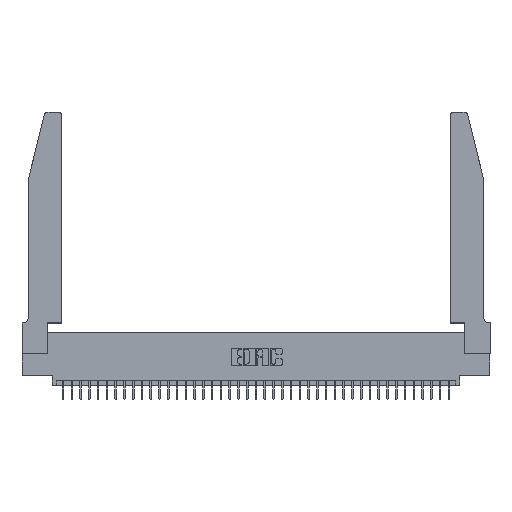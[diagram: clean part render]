
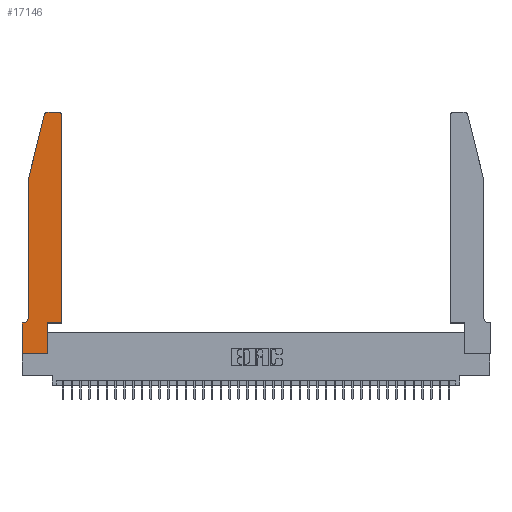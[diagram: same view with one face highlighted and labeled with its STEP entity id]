
A CAD part, top view. The second image highlights one B-rep face of the part: STEP entity #17146.
In plain terms, the highlighted planar face has unit normal (0, 0, 1).
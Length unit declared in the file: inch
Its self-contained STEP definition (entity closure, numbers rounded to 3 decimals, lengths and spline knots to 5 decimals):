
#1031 = EDGE_CURVE ( 'NONE', #5443, #14733, #7668, .T. ) ;
#1682 = ORIENTED_EDGE ( 'NONE', *, *, #4806, .T. ) ;
#1684 = DIRECTION ( 'NONE',  ( -1., 0., 0. ) ) ;
#2002 = AXIS2_PLACEMENT_3D ( 'NONE', #31600, #16380, #37752 ) ;
#3697 = CARTESIAN_POINT ( 'NONE',  ( 0.4505, 2.72, 0.37 ) ) ;
#4222 = CIRCLE ( 'NONE', #11011, 0.03 ) ;
#4514 = VERTEX_POINT ( 'NONE', #37365 ) ;
#4765 = EDGE_CURVE ( 'NONE', #20373, #31066, #15623, .T. ) ;
#4806 = EDGE_CURVE ( 'NONE', #36230, #12499, #21822, .T. ) ;
#4904 = CARTESIAN_POINT ( 'NONE',  ( 0.2865, 0.35, 0.37 ) ) ;
#4975 = CARTESIAN_POINT ( 'NONE',  ( 0.0055, 0.35, 0.37 ) ) ;
#5207 = DIRECTION ( 'NONE',  ( 0., -1., 0. ) ) ;
#5320 = LINE ( 'NONE', #6671, #22719 ) ;
#5443 = VERTEX_POINT ( 'NONE', #14033 ) ;
#5752 = EDGE_CURVE ( 'NONE', #4514, #20373, #5320, .T. ) ;
#5785 = AXIS2_PLACEMENT_3D ( 'NONE', #25825, #28760, #36079 ) ;
#6391 = DIRECTION ( 'NONE',  ( 0., 0., 1. ) ) ;
#6575 = ORIENTED_EDGE ( 'NONE', *, *, #12706, .T. ) ;
#6606 = LINE ( 'NONE', #24565, #22051 ) ;
#6671 = CARTESIAN_POINT ( 'NONE',  ( 0.2865, 0.35, 0.37 ) ) ;
#6973 = AXIS2_PLACEMENT_3D ( 'NONE', #29463, #11096, #32528 ) ;
#7668 = CIRCLE ( 'NONE', #5785, 0.07 ) ;
#7837 = CARTESIAN_POINT ( 'NONE',  ( 0.0755, 0.35, 0.37 ) ) ;
#9509 = LINE ( 'NONE', #7837, #15807 ) ;
#9516 = ORIENTED_EDGE ( 'NONE', *, *, #16183, .T. ) ;
#9641 = VERTEX_POINT ( 'NONE', #30494 ) ;
#9820 = VERTEX_POINT ( 'NONE', #3697 ) ;
#10236 = VECTOR ( 'NONE', #27787, 39.37008 ) ;
#10326 = EDGE_CURVE ( 'NONE', #31066, #9820, #20815, .T. ) ;
#10944 = ORIENTED_EDGE ( 'NONE', *, *, #12348, .T. ) ;
#11011 = AXIS2_PLACEMENT_3D ( 'NONE', #24871, #6391, #27922 ) ;
#11096 = DIRECTION ( 'NONE',  ( 0., 0., 1. ) ) ;
#11230 = LINE ( 'NONE', #21889, #10236 ) ;
#11442 = FACE_OUTER_BOUND ( 'NONE', #21088, .T. ) ;
#11488 = ORIENTED_EDGE ( 'NONE', *, *, #5752, .T. ) ;
#11703 = EDGE_CURVE ( 'NONE', #9820, #9641, #4222, .T. ) ;
#12258 = DIRECTION ( 'NONE',  ( 1., 0., 0. ) ) ;
#12348 = EDGE_CURVE ( 'NONE', #12499, #19050, #6606, .T. ) ;
#12444 = ORIENTED_EDGE ( 'NONE', *, *, #10326, .T. ) ;
#12495 = CARTESIAN_POINT ( 'NONE',  ( 0.284, 2.75, 0.37 ) ) ;
#12499 = VERTEX_POINT ( 'NONE', #25220 ) ;
#12706 = EDGE_CURVE ( 'NONE', #14733, #25466, #9509, .T. ) ;
#13267 = PLANE ( 'NONE',  #2002 ) ;
#13452 = VECTOR ( 'NONE', #12258, 39.37008 ) ;
#14033 = CARTESIAN_POINT ( 'NONE',  ( 0.0755, 0.42, 0.37 ) ) ;
#14384 = ORIENTED_EDGE ( 'NONE', *, *, #11703, .T. ) ;
#14646 = VECTOR ( 'NONE', #20123, 39.37008 ) ;
#14733 = VERTEX_POINT ( 'NONE', #4975 ) ;
#15494 = CARTESIAN_POINT ( 'NONE',  ( 0., 0., 0.37 ) ) ;
#15623 = LINE ( 'NONE', #29210, #14646 ) ;
#15807 = VECTOR ( 'NONE', #1684, 39.37008 ) ;
#16183 = EDGE_CURVE ( 'NONE', #21726, #4514, #38846, .T. ) ;
#16380 = DIRECTION ( 'NONE',  ( 0., 0., 1. ) ) ;
#17146 = ADVANCED_FACE ( 'NONE', ( #11442 ), #13267, .T. ) ;
#17246 = ORIENTED_EDGE ( 'NONE', *, *, #24270, .T. ) ;
#17452 = DIRECTION ( 'NONE',  ( 0., -1., 0. ) ) ;
#18832 = DIRECTION ( 'NONE',  ( 0., 1., 0. ) ) ;
#19050 = VERTEX_POINT ( 'NONE', #38569 ) ;
#19101 = EDGE_CURVE ( 'NONE', #25466, #21726, #32826, .T. ) ;
#19833 = VECTOR ( 'NONE', #18832, 39.37008 ) ;
#20123 = DIRECTION ( 'NONE',  ( 1., 0., 0. ) ) ;
#20373 = VERTEX_POINT ( 'NONE', #4904 ) ;
#20815 = LINE ( 'NONE', #24857, #19833 ) ;
#21065 = CARTESIAN_POINT ( 'NONE',  ( 0., 0., 0.37 ) ) ;
#21088 = EDGE_LOOP ( 'NONE', ( #17246, #1682, #10944, #35399, #36357, #6575, #33002, #9516, #11488, #35905, #12444, #14384 ) ) ;
#21726 = VERTEX_POINT ( 'NONE', #21065 ) ;
#21822 = CIRCLE ( 'NONE', #6973, 0.03 ) ;
#21889 = CARTESIAN_POINT ( 'NONE',  ( 0.2605, 2.75, 0.37 ) ) ;
#22051 = VECTOR ( 'NONE', #27614, 39.37008 ) ;
#22719 = VECTOR ( 'NONE', #28188, 39.37008 ) ;
#23301 = EDGE_CURVE ( 'NONE', #19050, #5443, #35737, .T. ) ;
#23736 = CARTESIAN_POINT ( 'NONE',  ( 0.0755, 2., 0.37 ) ) ;
#24270 = EDGE_CURVE ( 'NONE', #9641, #36230, #11230, .T. ) ;
#24565 = CARTESIAN_POINT ( 'NONE',  ( 0.0755, 2., 0.37 ) ) ;
#24857 = CARTESIAN_POINT ( 'NONE',  ( 0.4505, 0.35, 0.37 ) ) ;
#24871 = CARTESIAN_POINT ( 'NONE',  ( 0.4205, 2.72, 0.37 ) ) ;
#25220 = CARTESIAN_POINT ( 'NONE',  ( 0.25487, 2.72718, 0.37 ) ) ;
#25466 = VERTEX_POINT ( 'NONE', #33051 ) ;
#25825 = CARTESIAN_POINT ( 'NONE',  ( 0.0055, 0.42, 0.37 ) ) ;
#27614 = DIRECTION ( 'NONE',  ( -0.239, -0.971, 0. ) ) ;
#27787 = DIRECTION ( 'NONE',  ( -1., 0., 0. ) ) ;
#27922 = DIRECTION ( 'NONE',  ( 1., 0., 0. ) ) ;
#28188 = DIRECTION ( 'NONE',  ( 0., 1., 0. ) ) ;
#28760 = DIRECTION ( 'NONE',  ( 0., 0., -1. ) ) ;
#29210 = CARTESIAN_POINT ( 'NONE',  ( 0.4505, 0.35, 0.37 ) ) ;
#29463 = CARTESIAN_POINT ( 'NONE',  ( 0.284, 2.72, 0.37 ) ) ;
#30494 = CARTESIAN_POINT ( 'NONE',  ( 0.4205, 2.75, 0.37 ) ) ;
#30913 = VECTOR ( 'NONE', #17452, 39.37008 ) ;
#31066 = VERTEX_POINT ( 'NONE', #38863 ) ;
#31600 = CARTESIAN_POINT ( 'NONE',  ( 0., 0.35, 0.37 ) ) ;
#32528 = DIRECTION ( 'NONE',  ( 1., 0., 0. ) ) ;
#32776 = CARTESIAN_POINT ( 'NONE',  ( 0., 0., 0.37 ) ) ;
#32826 = LINE ( 'NONE', #32776, #30913 ) ;
#33002 = ORIENTED_EDGE ( 'NONE', *, *, #19101, .T. ) ;
#33051 = CARTESIAN_POINT ( 'NONE',  ( 0., 0.35, 0.37 ) ) ;
#35399 = ORIENTED_EDGE ( 'NONE', *, *, #23301, .T. ) ;
#35737 = LINE ( 'NONE', #23736, #36690 ) ;
#35905 = ORIENTED_EDGE ( 'NONE', *, *, #4765, .T. ) ;
#36079 = DIRECTION ( 'NONE',  ( -1., 0., 0. ) ) ;
#36230 = VERTEX_POINT ( 'NONE', #12495 ) ;
#36357 = ORIENTED_EDGE ( 'NONE', *, *, #1031, .T. ) ;
#36690 = VECTOR ( 'NONE', #5207, 39.37008 ) ;
#37365 = CARTESIAN_POINT ( 'NONE',  ( 0.2865, 0., 0.37 ) ) ;
#37752 = DIRECTION ( 'NONE',  ( 1., 0., 0. ) ) ;
#38569 = CARTESIAN_POINT ( 'NONE',  ( 0.0755, 2., 0.37 ) ) ;
#38846 = LINE ( 'NONE', #15494, #13452 ) ;
#38863 = CARTESIAN_POINT ( 'NONE',  ( 0.4505, 0.35, 0.37 ) ) ;
